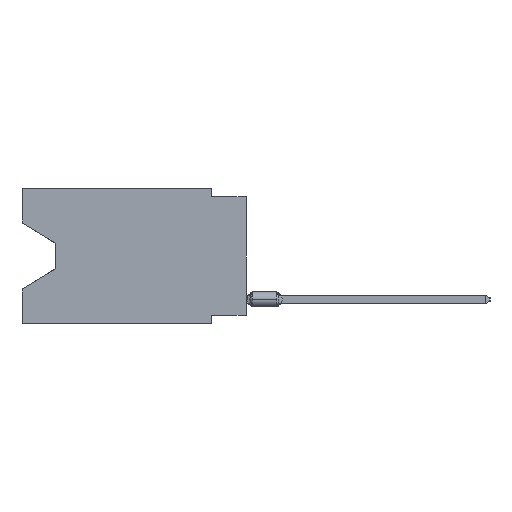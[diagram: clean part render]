
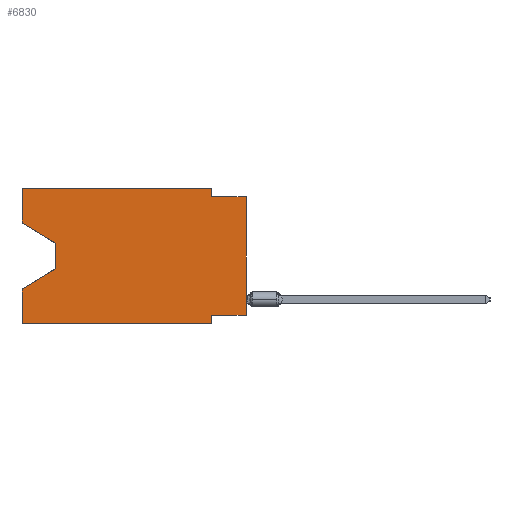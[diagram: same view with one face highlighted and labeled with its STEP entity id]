
A CAD part, left-side view. The second image highlights one B-rep face of the part: STEP entity #6830.
In plain terms, the highlighted planar face has unit normal (-1, 0, 0).
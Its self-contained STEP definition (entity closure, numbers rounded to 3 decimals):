
#332 = PLANE ( 'NONE',  #9730 ) ;
#1059 = CARTESIAN_POINT ( 'NONE',  ( 0., 16.383, -2.546 ) ) ;
#1137 = CARTESIAN_POINT ( 'NONE',  ( 0., 2.54, -9.906 ) ) ;
#1743 = EDGE_CURVE ( 'NONE', #21863, #10764, #19540, .T. ) ;
#2099 = CARTESIAN_POINT ( 'NONE',  ( 0., 16.383, -9.906 ) ) ;
#2437 = VERTEX_POINT ( 'NONE', #2719 ) ;
#2513 = ORIENTED_EDGE ( 'NONE', *, *, #6425, .F. ) ;
#2719 = CARTESIAN_POINT ( 'NONE',  ( 0., 16.383, -9.906 ) ) ;
#3142 = EDGE_CURVE ( 'NONE', #2437, #27081, #7175, .T. ) ;
#3213 = EDGE_CURVE ( 'NONE', #20261, #38472, #20263, .T. ) ;
#3245 = VERTEX_POINT ( 'NONE', #16422 ) ;
#3343 = VECTOR ( 'NONE', #24610, 1000. ) ;
#3663 = DIRECTION ( 'NONE',  ( 0., 0., -1. ) ) ;
#4023 = VECTOR ( 'NONE', #9287, 1000. ) ;
#4539 = VERTEX_POINT ( 'NONE', #1137 ) ;
#5179 = CARTESIAN_POINT ( 'NONE',  ( 0., 2.54, 0. ) ) ;
#6186 = VECTOR ( 'NONE', #13925, 1000. ) ;
#6248 = EDGE_CURVE ( 'NONE', #44849, #15529, #26700, .T. ) ;
#6260 = VERTEX_POINT ( 'NONE', #1059 ) ;
#6307 = CARTESIAN_POINT ( 'NONE',  ( 0., 0., -0.635 ) ) ;
#6425 = EDGE_CURVE ( 'NONE', #6827, #3245, #16307, .T. ) ;
#6827 = VERTEX_POINT ( 'NONE', #12615 ) ;
#6830 = ADVANCED_FACE ( 'NONE', ( #33354 ), #332, .F. ) ;
#7051 = CARTESIAN_POINT ( 'NONE',  ( 0., 0., 0. ) ) ;
#7175 = LINE ( 'NONE', #36367, #50412 ) ;
#7994 = VECTOR ( 'NONE', #10569, 1000. ) ;
#8516 = DIRECTION ( 'NONE',  ( 0., 0., -1. ) ) ;
#8784 = VECTOR ( 'NONE', #23111, 1000. ) ;
#9287 = DIRECTION ( 'NONE',  ( 0., 0., -1. ) ) ;
#9327 = VECTOR ( 'NONE', #14150, 1000. ) ;
#9730 = AXIS2_PLACEMENT_3D ( 'NONE', #50741, #12875, #8516 ) ;
#10341 = DIRECTION ( 'NONE',  ( 0., 0., 1. ) ) ;
#10569 = DIRECTION ( 'NONE',  ( 0., -1., 0. ) ) ;
#10764 = VERTEX_POINT ( 'NONE', #12219 ) ;
#10800 = VECTOR ( 'NONE', #24053, 1000. ) ;
#11145 = ORIENTED_EDGE ( 'NONE', *, *, #13932, .T. ) ;
#12219 = CARTESIAN_POINT ( 'NONE',  ( 0., 13.97, -5.893 ) ) ;
#12615 = CARTESIAN_POINT ( 'NONE',  ( 0., 16.383, 0. ) ) ;
#12875 = DIRECTION ( 'NONE',  ( 1., 0., 0. ) ) ;
#13865 = CARTESIAN_POINT ( 'NONE',  ( 0., 0., -9.271 ) ) ;
#13925 = DIRECTION ( 'NONE',  ( 0., 0., 1. ) ) ;
#13932 = EDGE_CURVE ( 'NONE', #44849, #38472, #52298, .T. ) ;
#14150 = DIRECTION ( 'NONE',  ( 0., 0.855, -0.519 ) ) ;
#15462 = ORIENTED_EDGE ( 'NONE', *, *, #3142, .F. ) ;
#15529 = VERTEX_POINT ( 'NONE', #29765 ) ;
#15747 = LINE ( 'NONE', #2099, #7994 ) ;
#16165 = CARTESIAN_POINT ( 'NONE',  ( 0., 0., -0.635 ) ) ;
#16307 = LINE ( 'NONE', #17110, #27070 ) ;
#16422 = CARTESIAN_POINT ( 'NONE',  ( 0., 2.54, 0. ) ) ;
#16494 = VECTOR ( 'NONE', #10341, 1000. ) ;
#17110 = CARTESIAN_POINT ( 'NONE',  ( 0., 16.383, 0. ) ) ;
#17191 = LINE ( 'NONE', #30532, #9327 ) ;
#18865 = LINE ( 'NONE', #48001, #6186 ) ;
#19270 = VECTOR ( 'NONE', #34884, 1000. ) ;
#19540 = LINE ( 'NONE', #41031, #49311 ) ;
#20261 = VERTEX_POINT ( 'NONE', #26965 ) ;
#20263 = LINE ( 'NONE', #16165, #3343 ) ;
#20928 = DIRECTION ( 'NONE',  ( 0., -1., 0. ) ) ;
#21863 = VERTEX_POINT ( 'NONE', #51730 ) ;
#23111 = DIRECTION ( 'NONE',  ( 0., -0.855, -0.519 ) ) ;
#24053 = DIRECTION ( 'NONE',  ( 0., 0., -1. ) ) ;
#24610 = DIRECTION ( 'NONE',  ( 0., -1., 0. ) ) ;
#26530 = CARTESIAN_POINT ( 'NONE',  ( 0., 16.383, -7.36 ) ) ;
#26700 = LINE ( 'NONE', #13865, #19270 ) ;
#26965 = CARTESIAN_POINT ( 'NONE',  ( 0., 2.54, -0.635 ) ) ;
#27070 = VECTOR ( 'NONE', #20928, 1000. ) ;
#27081 = VERTEX_POINT ( 'NONE', #26530 ) ;
#28113 = ORIENTED_EDGE ( 'NONE', *, *, #38523, .F. ) ;
#28575 = EDGE_CURVE ( 'NONE', #3245, #20261, #30268, .T. ) ;
#29168 = EDGE_CURVE ( 'NONE', #10764, #27081, #17191, .T. ) ;
#29765 = CARTESIAN_POINT ( 'NONE',  ( 0., 2.54, -9.271 ) ) ;
#30268 = LINE ( 'NONE', #5179, #4023 ) ;
#30532 = CARTESIAN_POINT ( 'NONE',  ( 0., 13.97, -5.893 ) ) ;
#30969 = ORIENTED_EDGE ( 'NONE', *, *, #1743, .T. ) ;
#32249 = LINE ( 'NONE', #49617, #10800 ) ;
#33354 = FACE_OUTER_BOUND ( 'NONE', #37406, .T. ) ;
#34183 = EDGE_CURVE ( 'NONE', #2437, #4539, #15747, .T. ) ;
#34884 = DIRECTION ( 'NONE',  ( 0., 1., 0. ) ) ;
#35015 = EDGE_CURVE ( 'NONE', #6260, #6827, #18865, .T. ) ;
#35065 = ORIENTED_EDGE ( 'NONE', *, *, #34183, .T. ) ;
#36367 = CARTESIAN_POINT ( 'NONE',  ( 0., 16.383, 0. ) ) ;
#36989 = ORIENTED_EDGE ( 'NONE', *, *, #29168, .T. ) ;
#37406 = EDGE_LOOP ( 'NONE', ( #40799, #30969, #36989, #15462, #35065, #28113, #42914, #11145, #38203, #38201, #2513, #53012 ) ) ;
#38201 = ORIENTED_EDGE ( 'NONE', *, *, #28575, .F. ) ;
#38203 = ORIENTED_EDGE ( 'NONE', *, *, #3213, .F. ) ;
#38472 = VERTEX_POINT ( 'NONE', #6307 ) ;
#38523 = EDGE_CURVE ( 'NONE', #15529, #4539, #32249, .T. ) ;
#40799 = ORIENTED_EDGE ( 'NONE', *, *, #46562, .T. ) ;
#41031 = CARTESIAN_POINT ( 'NONE',  ( 0., 13.97, -4.013 ) ) ;
#42914 = ORIENTED_EDGE ( 'NONE', *, *, #6248, .F. ) ;
#44849 = VERTEX_POINT ( 'NONE', #49678 ) ;
#46562 = EDGE_CURVE ( 'NONE', #6260, #21863, #48980, .T. ) ;
#48001 = CARTESIAN_POINT ( 'NONE',  ( 0., 16.383, 0. ) ) ;
#48440 = CARTESIAN_POINT ( 'NONE',  ( 0., 16.383, -2.546 ) ) ;
#48980 = LINE ( 'NONE', #48440, #8784 ) ;
#49311 = VECTOR ( 'NONE', #3663, 1000. ) ;
#49617 = CARTESIAN_POINT ( 'NONE',  ( 0., 2.54, -9.906 ) ) ;
#49678 = CARTESIAN_POINT ( 'NONE',  ( 0., 0., -9.271 ) ) ;
#50412 = VECTOR ( 'NONE', #52963, 1000. ) ;
#50741 = CARTESIAN_POINT ( 'NONE',  ( 0., 16.383, 0. ) ) ;
#51730 = CARTESIAN_POINT ( 'NONE',  ( 0., 13.97, -4.013 ) ) ;
#52298 = LINE ( 'NONE', #7051, #16494 ) ;
#52963 = DIRECTION ( 'NONE',  ( 0., 0., 1. ) ) ;
#53012 = ORIENTED_EDGE ( 'NONE', *, *, #35015, .F. ) ;
